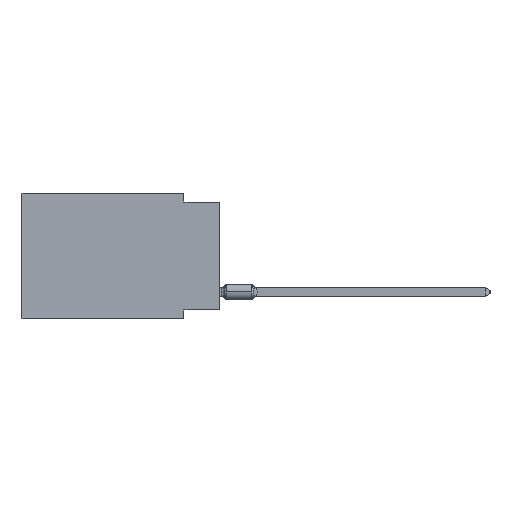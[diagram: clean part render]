
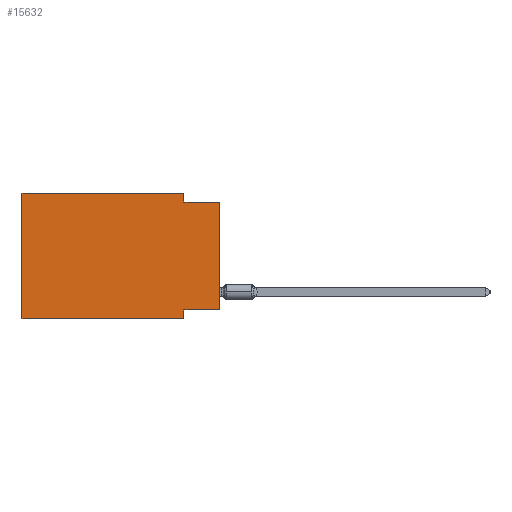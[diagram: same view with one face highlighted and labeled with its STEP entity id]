
A CAD part, left-side view. The second image highlights one B-rep face of the part: STEP entity #15632.
In plain terms, the highlighted planar face has unit normal (-1, 0, 0).
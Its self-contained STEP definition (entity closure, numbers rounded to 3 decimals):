
#1412 = CARTESIAN_POINT ( 'NONE',  ( 0., 2.54, -0.635 ) ) ;
#3578 = VERTEX_POINT ( 'NONE', #1412 ) ;
#3712 = VERTEX_POINT ( 'NONE', #23648 ) ;
#5006 = VERTEX_POINT ( 'NONE', #6035 ) ;
#6035 = CARTESIAN_POINT ( 'NONE',  ( 0., 2.54, -8.89 ) ) ;
#9505 = LINE ( 'NONE', #98252, #116216 ) ;
#10238 = EDGE_CURVE ( 'NONE', #93508, #94947, #100529, .T. ) ;
#10338 = DIRECTION ( 'NONE',  ( 0., 0., -1. ) ) ;
#11232 = DIRECTION ( 'NONE',  ( 0., 0., 1. ) ) ;
#11248 = LINE ( 'NONE', #101177, #54511 ) ;
#12294 = ORIENTED_EDGE ( 'NONE', *, *, #88752, .F. ) ;
#15632 = ADVANCED_FACE ( 'NONE', ( #99704 ), #80884, .F. ) ;
#15918 = CARTESIAN_POINT ( 'NONE',  ( 0., 0., -8.255 ) ) ;
#20365 = ORIENTED_EDGE ( 'NONE', *, *, #59059, .F. ) ;
#20710 = VERTEX_POINT ( 'NONE', #115295 ) ;
#22702 = CARTESIAN_POINT ( 'NONE',  ( 0., 2.54, -8.89 ) ) ;
#23648 = CARTESIAN_POINT ( 'NONE',  ( 0., 2.54, 0. ) ) ;
#23936 = DIRECTION ( 'NONE',  ( 0., 0., -1. ) ) ;
#24966 = VECTOR ( 'NONE', #23936, 1000. ) ;
#27506 = EDGE_LOOP ( 'NONE', ( #39074, #20365, #53859, #58788, #12294, #36778, #79907, #113412 ) ) ;
#29763 = EDGE_CURVE ( 'NONE', #93508, #94882, #54488, .T. ) ;
#30670 = CARTESIAN_POINT ( 'NONE',  ( 0., 0., -0.635 ) ) ;
#36778 = ORIENTED_EDGE ( 'NONE', *, *, #76555, .T. ) ;
#37140 = DIRECTION ( 'NONE',  ( 0., -1., 0. ) ) ;
#39074 = ORIENTED_EDGE ( 'NONE', *, *, #10238, .T. ) ;
#40342 = LINE ( 'NONE', #22702, #93146 ) ;
#44809 = EDGE_CURVE ( 'NONE', #20710, #3712, #11248, .T. ) ;
#46477 = DIRECTION ( 'NONE',  ( 0., 0., 1. ) ) ;
#46547 = DIRECTION ( 'NONE',  ( 0., -1., 0. ) ) ;
#50534 = VERTEX_POINT ( 'NONE', #94946 ) ;
#53859 = ORIENTED_EDGE ( 'NONE', *, *, #71337, .F. ) ;
#54488 = LINE ( 'NONE', #71563, #112156 ) ;
#54511 = VECTOR ( 'NONE', #46547, 1000. ) ;
#57601 = CARTESIAN_POINT ( 'NONE',  ( 0., 13.97, 0. ) ) ;
#58788 = ORIENTED_EDGE ( 'NONE', *, *, #44809, .F. ) ;
#59059 = EDGE_CURVE ( 'NONE', #3578, #94947, #9505, .T. ) ;
#63293 = DIRECTION ( 'NONE',  ( 0., 1., 0. ) ) ;
#67420 = LINE ( 'NONE', #77407, #24966 ) ;
#70852 = VECTOR ( 'NONE', #11232, 1000. ) ;
#71337 = EDGE_CURVE ( 'NONE', #3712, #3578, #67420, .T. ) ;
#71563 = CARTESIAN_POINT ( 'NONE',  ( 0., 0., -8.255 ) ) ;
#73396 = LINE ( 'NONE', #107558, #82930 ) ;
#74974 = DIRECTION ( 'NONE',  ( 0., 0., -1. ) ) ;
#76383 = LINE ( 'NONE', #57601, #70852 ) ;
#76555 = EDGE_CURVE ( 'NONE', #50534, #5006, #73396, .T. ) ;
#77407 = CARTESIAN_POINT ( 'NONE',  ( 0., 2.54, 0. ) ) ;
#79907 = ORIENTED_EDGE ( 'NONE', *, *, #116091, .F. ) ;
#80884 = PLANE ( 'NONE',  #101535 ) ;
#82930 = VECTOR ( 'NONE', #101018, 1000. ) ;
#88752 = EDGE_CURVE ( 'NONE', #50534, #20710, #76383, .T. ) ;
#90847 = CARTESIAN_POINT ( 'NONE',  ( 0., 13.97, 0. ) ) ;
#93146 = VECTOR ( 'NONE', #74974, 1000. ) ;
#93508 = VERTEX_POINT ( 'NONE', #15918 ) ;
#94094 = VECTOR ( 'NONE', #46477, 1000. ) ;
#94882 = VERTEX_POINT ( 'NONE', #99988 ) ;
#94946 = CARTESIAN_POINT ( 'NONE',  ( 0., 13.97, -8.89 ) ) ;
#94947 = VERTEX_POINT ( 'NONE', #30670 ) ;
#98252 = CARTESIAN_POINT ( 'NONE',  ( 0., 0., -0.635 ) ) ;
#99704 = FACE_OUTER_BOUND ( 'NONE', #27506, .T. ) ;
#99988 = CARTESIAN_POINT ( 'NONE',  ( 0., 2.54, -8.255 ) ) ;
#100529 = LINE ( 'NONE', #107212, #94094 ) ;
#101018 = DIRECTION ( 'NONE',  ( 0., -1., 0. ) ) ;
#101177 = CARTESIAN_POINT ( 'NONE',  ( 0., 13.97, 0. ) ) ;
#101535 = AXIS2_PLACEMENT_3D ( 'NONE', #90847, #107376, #10338 ) ;
#107212 = CARTESIAN_POINT ( 'NONE',  ( 0., 0., 0. ) ) ;
#107376 = DIRECTION ( 'NONE',  ( 1., 0., 0. ) ) ;
#107558 = CARTESIAN_POINT ( 'NONE',  ( 0., 13.97, -8.89 ) ) ;
#112156 = VECTOR ( 'NONE', #63293, 1000. ) ;
#113412 = ORIENTED_EDGE ( 'NONE', *, *, #29763, .F. ) ;
#115295 = CARTESIAN_POINT ( 'NONE',  ( 0., 13.97, 0. ) ) ;
#116091 = EDGE_CURVE ( 'NONE', #94882, #5006, #40342, .T. ) ;
#116216 = VECTOR ( 'NONE', #37140, 1000. ) ;
